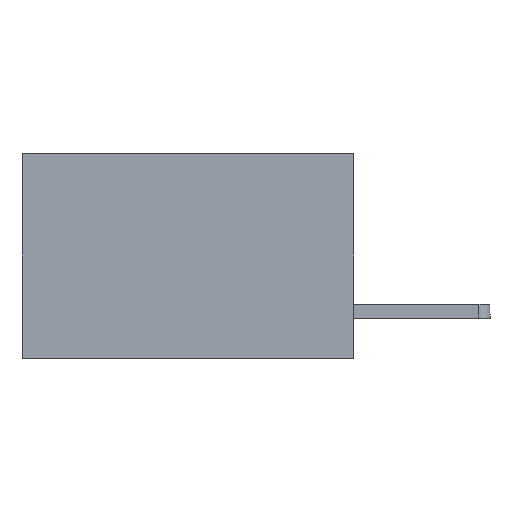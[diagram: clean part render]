
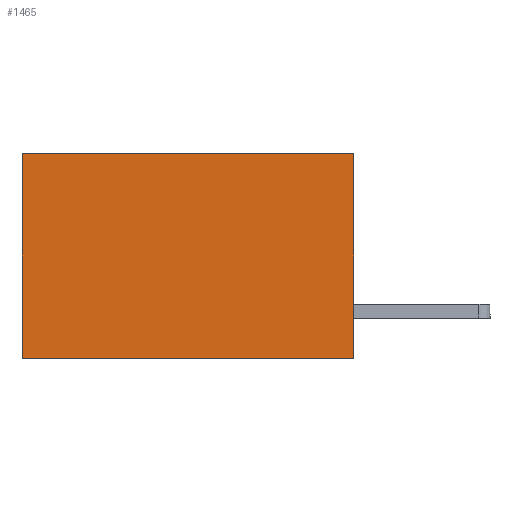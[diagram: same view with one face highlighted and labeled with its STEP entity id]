
A CAD part, left-side view. The second image highlights one B-rep face of the part: STEP entity #1465.
In plain terms, the highlighted planar face has unit normal (-1, 0, 0).
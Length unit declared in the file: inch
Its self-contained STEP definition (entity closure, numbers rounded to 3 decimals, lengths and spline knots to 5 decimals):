
#402 = ORIENTED_EDGE ( 'NONE', *, *, #2390, .T. ) ;
#1119 = VECTOR ( 'NONE', #2181, 39.37008 ) ;
#1306 = LINE ( 'NONE', #6177, #10435 ) ;
#1404 = LINE ( 'NONE', #2375, #1119 ) ;
#1465 = ADVANCED_FACE ( 'NONE', ( #7852 ), #4623, .F. ) ;
#1522 = VERTEX_POINT ( 'NONE', #9451 ) ;
#1608 = LINE ( 'NONE', #5483, #10724 ) ;
#1937 = DIRECTION ( 'NONE',  ( 0., 0., -1. ) ) ;
#2099 = VERTEX_POINT ( 'NONE', #4730 ) ;
#2181 = DIRECTION ( 'NONE',  ( 0., 0., -1. ) ) ;
#2375 = CARTESIAN_POINT ( 'NONE',  ( 0.2875, 0., 0. ) ) ;
#2390 = EDGE_CURVE ( 'NONE', #8330, #1522, #1608, .T. ) ;
#2716 = DIRECTION ( 'NONE',  ( 0., 1., 0. ) ) ;
#2846 = CARTESIAN_POINT ( 'NONE',  ( 0.2875, 0., 0. ) ) ;
#2858 = CARTESIAN_POINT ( 'NONE',  ( 0.2875, 0., -0.37 ) ) ;
#2985 = AXIS2_PLACEMENT_3D ( 'NONE', #2846, #7277, #1937 ) ;
#3116 = EDGE_CURVE ( 'NONE', #3496, #2099, #10013, .T. ) ;
#3227 = CARTESIAN_POINT ( 'NONE',  ( 0.2875, 0., -0.37 ) ) ;
#3496 = VERTEX_POINT ( 'NONE', #3227 ) ;
#4623 = PLANE ( 'NONE',  #2985 ) ;
#4730 = CARTESIAN_POINT ( 'NONE',  ( 0.2875, 0.6, -0.37 ) ) ;
#5049 = EDGE_CURVE ( 'NONE', #1522, #2099, #1306, .T. ) ;
#5483 = CARTESIAN_POINT ( 'NONE',  ( 0.2875, 0., 0. ) ) ;
#6006 = DIRECTION ( 'NONE',  ( 0., 0., -1. ) ) ;
#6177 = CARTESIAN_POINT ( 'NONE',  ( 0.2875, 0.6, 0. ) ) ;
#6679 = ORIENTED_EDGE ( 'NONE', *, *, #7433, .F. ) ;
#6905 = ORIENTED_EDGE ( 'NONE', *, *, #5049, .T. ) ;
#7277 = DIRECTION ( 'NONE',  ( 1., 0., 0. ) ) ;
#7433 = EDGE_CURVE ( 'NONE', #8330, #3496, #1404, .T. ) ;
#7435 = VECTOR ( 'NONE', #7471, 39.37008 ) ;
#7471 = DIRECTION ( 'NONE',  ( 0., 1., 0. ) ) ;
#7730 = EDGE_LOOP ( 'NONE', ( #6905, #9548, #6679, #402 ) ) ;
#7852 = FACE_OUTER_BOUND ( 'NONE', #7730, .T. ) ;
#8011 = CARTESIAN_POINT ( 'NONE',  ( 0.2875, 0., 0. ) ) ;
#8330 = VERTEX_POINT ( 'NONE', #8011 ) ;
#9451 = CARTESIAN_POINT ( 'NONE',  ( 0.2875, 0.6, 0. ) ) ;
#9548 = ORIENTED_EDGE ( 'NONE', *, *, #3116, .F. ) ;
#10013 = LINE ( 'NONE', #2858, #7435 ) ;
#10435 = VECTOR ( 'NONE', #6006, 39.37008 ) ;
#10724 = VECTOR ( 'NONE', #2716, 39.37008 ) ;
